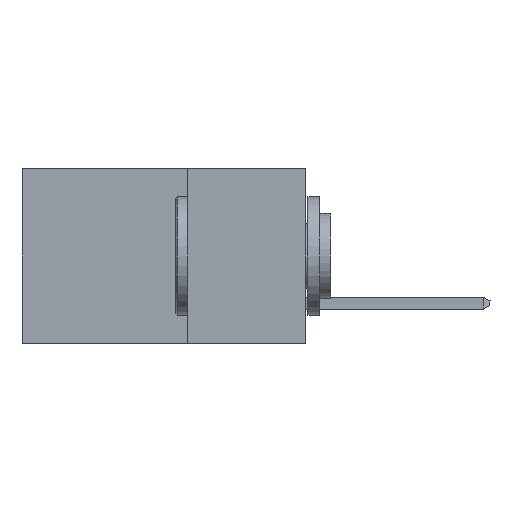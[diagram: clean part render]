
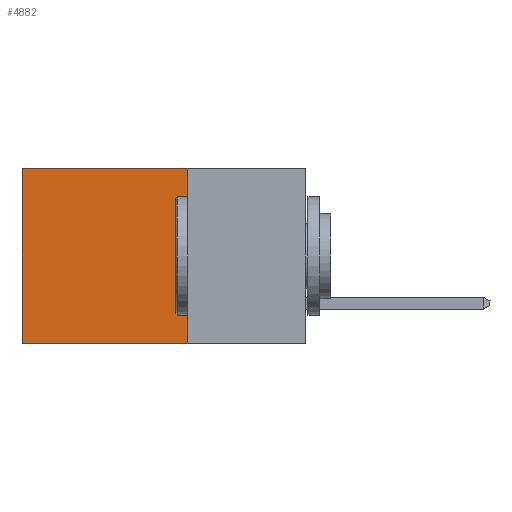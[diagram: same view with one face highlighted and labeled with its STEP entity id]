
A CAD part, left-side view. The second image highlights one B-rep face of the part: STEP entity #4882.
In plain terms, the highlighted planar face has unit normal (-1, 0, 0).
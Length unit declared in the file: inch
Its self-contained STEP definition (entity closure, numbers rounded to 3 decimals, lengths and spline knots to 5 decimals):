
#1027 = PLANE ( 'NONE',  #28059 ) ;
#2302 = VECTOR ( 'NONE', #27093, 39.37008 ) ;
#2560 = LINE ( 'NONE', #30135, #25284 ) ;
#3616 = LINE ( 'NONE', #31805, #15596 ) ;
#4081 = VERTEX_POINT ( 'NONE', #11015 ) ;
#4653 = CARTESIAN_POINT ( 'NONE',  ( 0.298, 0.25, 0. ) ) ;
#4882 = ADVANCED_FACE ( 'NONE', ( #17918 ), #1027, .F. ) ;
#7340 = EDGE_LOOP ( 'NONE', ( #23787, #10753, #31884, #27478 ) ) ;
#9716 = DIRECTION ( 'NONE',  ( 0., 1., 0. ) ) ;
#10746 = VERTEX_POINT ( 'NONE', #17129 ) ;
#10753 = ORIENTED_EDGE ( 'NONE', *, *, #22402, .F. ) ;
#11015 = CARTESIAN_POINT ( 'NONE',  ( 0.298, 0.25, -0.37 ) ) ;
#13119 = CARTESIAN_POINT ( 'NONE',  ( 0.298, 0.25, 0. ) ) ;
#13857 = EDGE_CURVE ( 'NONE', #22285, #10746, #2560, .T. ) ;
#14721 = VERTEX_POINT ( 'NONE', #13119 ) ;
#15596 = VECTOR ( 'NONE', #19630, 39.37008 ) ;
#17129 = CARTESIAN_POINT ( 'NONE',  ( 0.298, 0.6, -0.37 ) ) ;
#17822 = LINE ( 'NONE', #4653, #31240 ) ;
#17918 = FACE_OUTER_BOUND ( 'NONE', #7340, .T. ) ;
#18137 = DIRECTION ( 'NONE',  ( 0., 0., -1. ) ) ;
#18287 = DIRECTION ( 'NONE',  ( 1., 0., 0. ) ) ;
#19017 = EDGE_CURVE ( 'NONE', #14721, #4081, #30030, .T. ) ;
#19630 = DIRECTION ( 'NONE',  ( 0., 1., 0. ) ) ;
#22183 = CARTESIAN_POINT ( 'NONE',  ( 0.298, 0.6, 0. ) ) ;
#22285 = VERTEX_POINT ( 'NONE', #22183 ) ;
#22402 = EDGE_CURVE ( 'NONE', #4081, #10746, #3616, .T. ) ;
#23416 = EDGE_CURVE ( 'NONE', #14721, #22285, #17822, .T. ) ;
#23787 = ORIENTED_EDGE ( 'NONE', *, *, #13857, .T. ) ;
#25284 = VECTOR ( 'NONE', #18137, 39.37008 ) ;
#26114 = DIRECTION ( 'NONE',  ( 0., 0., -1. ) ) ;
#27093 = DIRECTION ( 'NONE',  ( 0., 0., -1. ) ) ;
#27203 = CARTESIAN_POINT ( 'NONE',  ( 0.298, 0.25, 0. ) ) ;
#27478 = ORIENTED_EDGE ( 'NONE', *, *, #23416, .T. ) ;
#28059 = AXIS2_PLACEMENT_3D ( 'NONE', #28263, #18287, #26114 ) ;
#28263 = CARTESIAN_POINT ( 'NONE',  ( 0.298, 0.25, 0. ) ) ;
#30030 = LINE ( 'NONE', #27203, #2302 ) ;
#30135 = CARTESIAN_POINT ( 'NONE',  ( 0.298, 0.6, 0. ) ) ;
#31240 = VECTOR ( 'NONE', #9716, 39.37008 ) ;
#31805 = CARTESIAN_POINT ( 'NONE',  ( 0.298, 0.25, -0.37 ) ) ;
#31884 = ORIENTED_EDGE ( 'NONE', *, *, #19017, .F. ) ;
